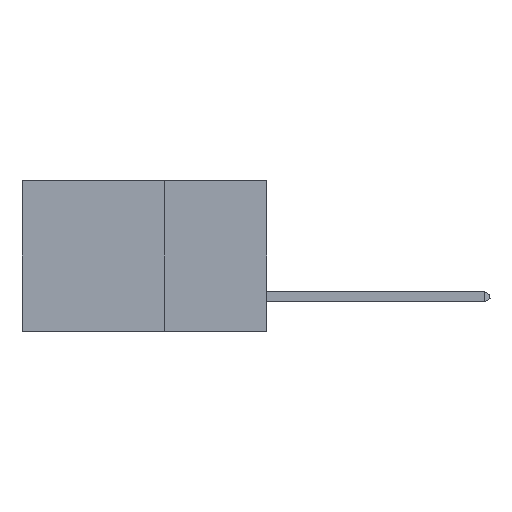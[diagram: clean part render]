
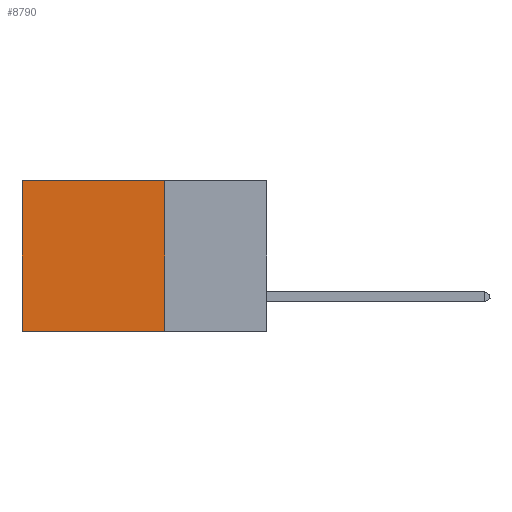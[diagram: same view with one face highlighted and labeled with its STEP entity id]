
A CAD part, left-side view. The second image highlights one B-rep face of the part: STEP entity #8790.
In plain terms, the highlighted planar face has unit normal (-1, 0, 0).
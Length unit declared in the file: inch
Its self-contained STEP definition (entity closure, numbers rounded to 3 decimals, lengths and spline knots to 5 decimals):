
#3682 = LINE ( 'NONE', #24422, #28409 ) ;
#4776 = AXIS2_PLACEMENT_3D ( 'NONE', #18153, #41593, #12935 ) ;
#5392 = CARTESIAN_POINT ( 'NONE',  ( 0.2875, 0.6, -0.37 ) ) ;
#7034 = ORIENTED_EDGE ( 'NONE', *, *, #27925, .F. ) ;
#7119 = DIRECTION ( 'NONE',  ( 0., 0., -1. ) ) ;
#7243 = EDGE_CURVE ( 'NONE', #11687, #13796, #33803, .T. ) ;
#8790 = ADVANCED_FACE ( 'NONE', ( #12176 ), #16064, .F. ) ;
#8800 = CARTESIAN_POINT ( 'NONE',  ( 0.2875, 0.6, 0. ) ) ;
#10187 = VECTOR ( 'NONE', #21657, 39.37008 ) ;
#11499 = CARTESIAN_POINT ( 'NONE',  ( 0.2875, 0.25, -0.37 ) ) ;
#11687 = VERTEX_POINT ( 'NONE', #8800 ) ;
#12176 = FACE_OUTER_BOUND ( 'NONE', #17652, .T. ) ;
#12935 = DIRECTION ( 'NONE',  ( 0., 0., -1. ) ) ;
#13796 = VERTEX_POINT ( 'NONE', #5392 ) ;
#14750 = CARTESIAN_POINT ( 'NONE',  ( 0.2875, 0.6, 0. ) ) ;
#16064 = PLANE ( 'NONE',  #4776 ) ;
#16199 = EDGE_CURVE ( 'NONE', #28191, #11687, #3682, .T. ) ;
#17252 = ORIENTED_EDGE ( 'NONE', *, *, #37772, .F. ) ;
#17652 = EDGE_LOOP ( 'NONE', ( #19464, #17252, #7034, #20747 ) ) ;
#18153 = CARTESIAN_POINT ( 'NONE',  ( 0.2875, 0.25, 0. ) ) ;
#18519 = VECTOR ( 'NONE', #31766, 39.37008 ) ;
#18920 = LINE ( 'NONE', #31207, #30971 ) ;
#19464 = ORIENTED_EDGE ( 'NONE', *, *, #7243, .T. ) ;
#20747 = ORIENTED_EDGE ( 'NONE', *, *, #16199, .T. ) ;
#21657 = DIRECTION ( 'NONE',  ( 0., 0., -1. ) ) ;
#22776 = LINE ( 'NONE', #11499, #18519 ) ;
#23173 = VERTEX_POINT ( 'NONE', #38619 ) ;
#24422 = CARTESIAN_POINT ( 'NONE',  ( 0.2875, 0.25, 0. ) ) ;
#27925 = EDGE_CURVE ( 'NONE', #28191, #23173, #18920, .T. ) ;
#27944 = DIRECTION ( 'NONE',  ( 0., 1., 0. ) ) ;
#28191 = VERTEX_POINT ( 'NONE', #34336 ) ;
#28409 = VECTOR ( 'NONE', #27944, 39.37008 ) ;
#30971 = VECTOR ( 'NONE', #7119, 39.37008 ) ;
#31207 = CARTESIAN_POINT ( 'NONE',  ( 0.2875, 0.25, 0. ) ) ;
#31766 = DIRECTION ( 'NONE',  ( 0., 1., 0. ) ) ;
#33803 = LINE ( 'NONE', #14750, #10187 ) ;
#34336 = CARTESIAN_POINT ( 'NONE',  ( 0.2875, 0.25, 0. ) ) ;
#37772 = EDGE_CURVE ( 'NONE', #23173, #13796, #22776, .T. ) ;
#38619 = CARTESIAN_POINT ( 'NONE',  ( 0.2875, 0.25, -0.37 ) ) ;
#41593 = DIRECTION ( 'NONE',  ( 1., 0., 0. ) ) ;
